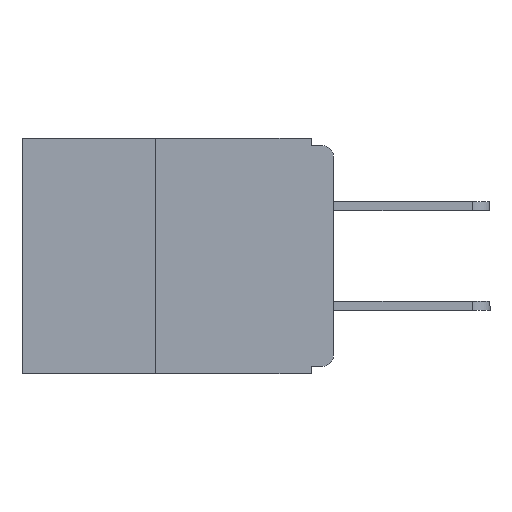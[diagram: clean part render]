
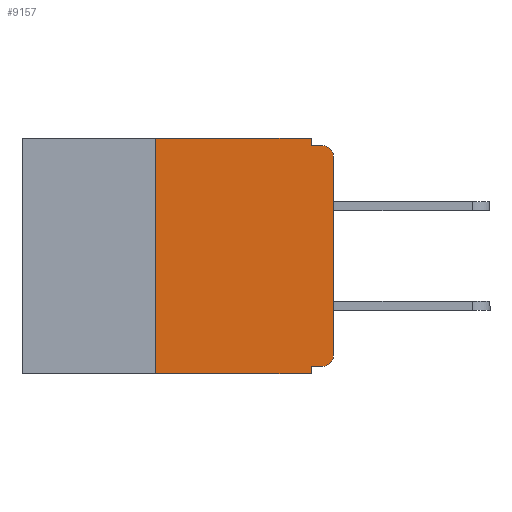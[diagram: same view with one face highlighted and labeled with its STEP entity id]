
A CAD part, left-side view. The second image highlights one B-rep face of the part: STEP entity #9157.
In plain terms, the highlighted planar face has unit normal (-1, 0, 0).
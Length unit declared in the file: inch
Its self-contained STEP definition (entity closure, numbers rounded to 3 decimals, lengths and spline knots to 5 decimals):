
#212 = VERTEX_POINT ( 'NONE', #3177 ) ;
#455 = CARTESIAN_POINT ( 'NONE',  ( 0., 0.031, -0.01 ) ) ;
#645 = LINE ( 'NONE', #3820, #16895 ) ;
#698 = VERTEX_POINT ( 'NONE', #14436 ) ;
#1116 = ORIENTED_EDGE ( 'NONE', *, *, #11581, .F. ) ;
#1368 = DIRECTION ( 'NONE',  ( 0., 0., -1. ) ) ;
#2073 = CARTESIAN_POINT ( 'NONE',  ( 0., 0.015, -0.305 ) ) ;
#2500 = ORIENTED_EDGE ( 'NONE', *, *, #8225, .T. ) ;
#3177 = CARTESIAN_POINT ( 'NONE',  ( 0., 0., -0.305 ) ) ;
#3642 = DIRECTION ( 'NONE',  ( 0., 0., 1. ) ) ;
#3820 = CARTESIAN_POINT ( 'NONE',  ( 0., 0., -0.32 ) ) ;
#3853 = CARTESIAN_POINT ( 'NONE',  ( 0., 0.031, -0.33 ) ) ;
#4316 = EDGE_CURVE ( 'NONE', #15523, #698, #16677, .T. ) ;
#4341 = DIRECTION ( 'NONE',  ( 0., 0., -1. ) ) ;
#4902 = CARTESIAN_POINT ( 'NONE',  ( 0., 0.031, 0. ) ) ;
#5508 = LINE ( 'NONE', #4902, #20987 ) ;
#5831 = VECTOR ( 'NONE', #1368, 39.37008 ) ;
#5870 = DIRECTION ( 'NONE',  ( 0., 0., -1. ) ) ;
#6238 = CARTESIAN_POINT ( 'NONE',  ( 0., 0.25, -0.33 ) ) ;
#6281 = VECTOR ( 'NONE', #14809, 39.37008 ) ;
#6423 = VECTOR ( 'NONE', #10639, 39.37008 ) ;
#6430 = CIRCLE ( 'NONE', #14421, 0.015 ) ;
#6866 = ORIENTED_EDGE ( 'NONE', *, *, #24443, .F. ) ;
#7084 = VECTOR ( 'NONE', #9839, 39.37008 ) ;
#7121 = DIRECTION ( 'NONE',  ( 0., 0., -1. ) ) ;
#8068 = CARTESIAN_POINT ( 'NONE',  ( 0., 0.25, -0.33 ) ) ;
#8225 = EDGE_CURVE ( 'NONE', #22995, #212, #6430, .T. ) ;
#8879 = LINE ( 'NONE', #8068, #26929 ) ;
#9157 = ADVANCED_FACE ( 'NONE', ( #15989 ), #12393, .F. ) ;
#9743 = ORIENTED_EDGE ( 'NONE', *, *, #27371, .T. ) ;
#9839 = DIRECTION ( 'NONE',  ( 0., -1., 0. ) ) ;
#10306 = AXIS2_PLACEMENT_3D ( 'NONE', #11050, #11008, #10955 ) ;
#10639 = DIRECTION ( 'NONE',  ( 0., 0., 1. ) ) ;
#10955 = DIRECTION ( 'NONE',  ( 0., 0., -1. ) ) ;
#11008 = DIRECTION ( 'NONE',  ( -1., 0., 0. ) ) ;
#11050 = CARTESIAN_POINT ( 'NONE',  ( 0., 0.015, -0.025 ) ) ;
#11581 = EDGE_CURVE ( 'NONE', #19004, #18587, #28252, .T. ) ;
#12084 = EDGE_CURVE ( 'NONE', #14987, #25860, #8879, .T. ) ;
#12262 = LINE ( 'NONE', #25891, #6423 ) ;
#12393 = PLANE ( 'NONE',  #27307 ) ;
#12581 = CARTESIAN_POINT ( 'NONE',  ( 0., 0.437, 0. ) ) ;
#12645 = DIRECTION ( 'NONE',  ( 0., 1., 0. ) ) ;
#12904 = LINE ( 'NONE', #25126, #7084 ) ;
#13985 = CARTESIAN_POINT ( 'NONE',  ( 0., 0.031, -0.32 ) ) ;
#14097 = CARTESIAN_POINT ( 'NONE',  ( 0., 0., -0.01 ) ) ;
#14421 = AXIS2_PLACEMENT_3D ( 'NONE', #2073, #17500, #4341 ) ;
#14436 = CARTESIAN_POINT ( 'NONE',  ( 0., 0.015, -0.01 ) ) ;
#14590 = CARTESIAN_POINT ( 'NONE',  ( 0., 0.031, -0.33 ) ) ;
#14809 = DIRECTION ( 'NONE',  ( 0., -1., 0. ) ) ;
#14987 = VERTEX_POINT ( 'NONE', #6238 ) ;
#15078 = VECTOR ( 'NONE', #20647, 39.37008 ) ;
#15523 = VERTEX_POINT ( 'NONE', #23169 ) ;
#15989 = FACE_OUTER_BOUND ( 'NONE', #26040, .T. ) ;
#16677 = CIRCLE ( 'NONE', #10306, 0.015 ) ;
#16895 = VECTOR ( 'NONE', #12645, 39.37008 ) ;
#17449 = EDGE_CURVE ( 'NONE', #212, #15523, #12262, .T. ) ;
#17500 = DIRECTION ( 'NONE',  ( -1., 0., 0. ) ) ;
#18341 = ORIENTED_EDGE ( 'NONE', *, *, #17449, .T. ) ;
#18587 = VERTEX_POINT ( 'NONE', #3853 ) ;
#18640 = LINE ( 'NONE', #12581, #6281 ) ;
#19004 = VERTEX_POINT ( 'NONE', #13985 ) ;
#19016 = DIRECTION ( 'NONE',  ( 1., 0., 0. ) ) ;
#19988 = CARTESIAN_POINT ( 'NONE',  ( 0., 0.25, 0. ) ) ;
#20315 = VERTEX_POINT ( 'NONE', #25304 ) ;
#20647 = DIRECTION ( 'NONE',  ( 0., -1., 0. ) ) ;
#20987 = VECTOR ( 'NONE', #7121, 39.37008 ) ;
#22599 = ORIENTED_EDGE ( 'NONE', *, *, #4316, .T. ) ;
#22628 = ORIENTED_EDGE ( 'NONE', *, *, #26065, .F. ) ;
#22995 = VERTEX_POINT ( 'NONE', #24662 ) ;
#23169 = CARTESIAN_POINT ( 'NONE',  ( 0., 0., -0.025 ) ) ;
#23298 = CARTESIAN_POINT ( 'NONE',  ( 0., 0.437, 0. ) ) ;
#23558 = ORIENTED_EDGE ( 'NONE', *, *, #27849, .F. ) ;
#23763 = EDGE_CURVE ( 'NONE', #25860, #20315, #18640, .T. ) ;
#23822 = ORIENTED_EDGE ( 'NONE', *, *, #23763, .F. ) ;
#24443 = EDGE_CURVE ( 'NONE', #22995, #19004, #645, .T. ) ;
#24662 = CARTESIAN_POINT ( 'NONE',  ( 0., 0.015, -0.32 ) ) ;
#24927 = ORIENTED_EDGE ( 'NONE', *, *, #12084, .F. ) ;
#25126 = CARTESIAN_POINT ( 'NONE',  ( 0., 0.437, -0.33 ) ) ;
#25304 = CARTESIAN_POINT ( 'NONE',  ( 0., 0.031, 0. ) ) ;
#25860 = VERTEX_POINT ( 'NONE', #19988 ) ;
#25891 = CARTESIAN_POINT ( 'NONE',  ( 0., 0., 0. ) ) ;
#26040 = EDGE_LOOP ( 'NONE', ( #18341, #22599, #22628, #23558, #23822, #24927, #9743, #1116, #6866, #2500 ) ) ;
#26065 = EDGE_CURVE ( 'NONE', #26608, #698, #27256, .T. ) ;
#26608 = VERTEX_POINT ( 'NONE', #455 ) ;
#26929 = VECTOR ( 'NONE', #3642, 39.37008 ) ;
#27256 = LINE ( 'NONE', #14097, #15078 ) ;
#27307 = AXIS2_PLACEMENT_3D ( 'NONE', #23298, #19016, #5870 ) ;
#27371 = EDGE_CURVE ( 'NONE', #14987, #18587, #12904, .T. ) ;
#27849 = EDGE_CURVE ( 'NONE', #20315, #26608, #5508, .T. ) ;
#28252 = LINE ( 'NONE', #14590, #5831 ) ;
